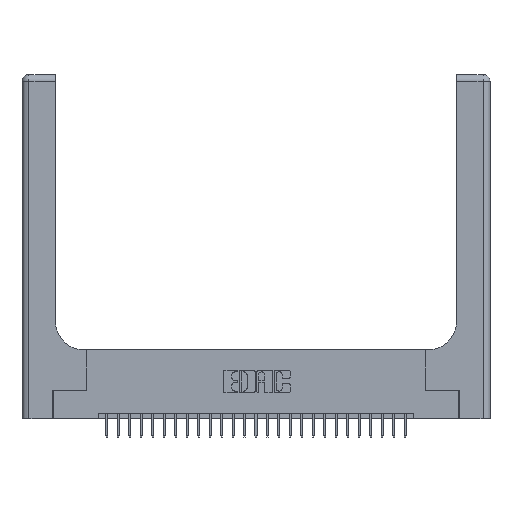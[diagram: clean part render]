
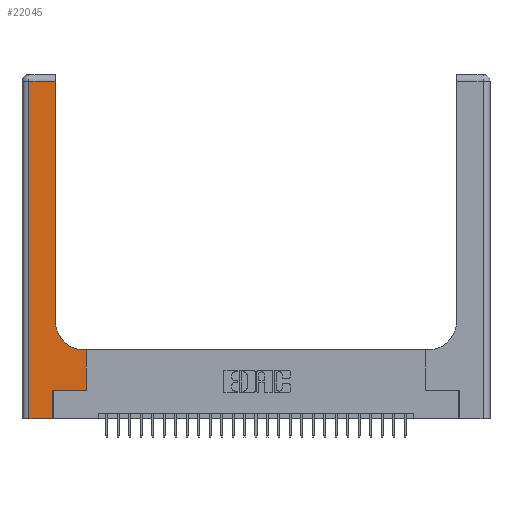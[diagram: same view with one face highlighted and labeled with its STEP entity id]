
A CAD part, top view. The second image highlights one B-rep face of the part: STEP entity #22045.
In plain terms, the highlighted planar face has unit normal (0, 0, 1).
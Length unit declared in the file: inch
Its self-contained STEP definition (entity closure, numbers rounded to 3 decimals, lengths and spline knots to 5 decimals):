
#95 = CARTESIAN_POINT ( 'NONE',  ( 0., 2.94, 0.37 ) ) ;
#157 = VECTOR ( 'NONE', #3752, 39.37008 ) ;
#340 = CARTESIAN_POINT ( 'NONE',  ( 0.5585, 0.6, 0.37 ) ) ;
#359 = EDGE_CURVE ( 'NONE', #14216, #27336, #12502, .T. ) ;
#906 = VERTEX_POINT ( 'NONE', #1702 ) ;
#1003 = ORIENTED_EDGE ( 'NONE', *, *, #15450, .T. ) ;
#1260 = AXIS2_PLACEMENT_3D ( 'NONE', #23808, #10776, #25950 ) ;
#1341 = CARTESIAN_POINT ( 'NONE',  ( 0.5415, 0.6, 0.37 ) ) ;
#1397 = ORIENTED_EDGE ( 'NONE', *, *, #9048, .T. ) ;
#1694 = CARTESIAN_POINT ( 'NONE',  ( 0.5585, 0.25, 0.37 ) ) ;
#1702 = CARTESIAN_POINT ( 'NONE',  ( 0.06, 2.94, 0.37 ) ) ;
#2161 = DIRECTION ( 'NONE',  ( -1., 0., 0. ) ) ;
#2397 = DIRECTION ( 'NONE',  ( -1., 0., 0. ) ) ;
#2763 = CARTESIAN_POINT ( 'NONE',  ( 0.06, 3., 0.37 ) ) ;
#2784 = VECTOR ( 'NONE', #6668, 39.37008 ) ;
#3312 = VERTEX_POINT ( 'NONE', #1694 ) ;
#3359 = VERTEX_POINT ( 'NONE', #10754 ) ;
#3545 = CARTESIAN_POINT ( 'NONE',  ( 0.2915, 2.94, 0.37 ) ) ;
#3582 = ORIENTED_EDGE ( 'NONE', *, *, #26707, .T. ) ;
#3752 = DIRECTION ( 'NONE',  ( 0., 1., 0. ) ) ;
#4565 = ORIENTED_EDGE ( 'NONE', *, *, #6245, .T. ) ;
#5023 = DIRECTION ( 'NONE',  ( 0., -1., 0. ) ) ;
#5375 = ORIENTED_EDGE ( 'NONE', *, *, #9801, .T. ) ;
#6245 = EDGE_CURVE ( 'NONE', #17112, #3359, #12211, .T. ) ;
#6668 = DIRECTION ( 'NONE',  ( 1., 0., 0. ) ) ;
#7651 = DIRECTION ( 'NONE',  ( 0., 1., 0. ) ) ;
#8170 = VERTEX_POINT ( 'NONE', #3545 ) ;
#8178 = EDGE_LOOP ( 'NONE', ( #24019, #5375, #8400, #12252, #4565, #1397, #3582, #14459, #1003 ) ) ;
#8400 = ORIENTED_EDGE ( 'NONE', *, *, #16380, .T. ) ;
#8518 = VECTOR ( 'NONE', #25451, 39.37008 ) ;
#8765 = LINE ( 'NONE', #19908, #2784 ) ;
#8846 = DIRECTION ( 'NONE',  ( 0., 0., -1. ) ) ;
#8853 = DIRECTION ( 'NONE',  ( 1., 0., 0. ) ) ;
#8907 = VERTEX_POINT ( 'NONE', #19254 ) ;
#9048 = EDGE_CURVE ( 'NONE', #3359, #3312, #8765, .T. ) ;
#9801 = EDGE_CURVE ( 'NONE', #8170, #906, #15629, .T. ) ;
#10754 = CARTESIAN_POINT ( 'NONE',  ( 0.269, 0.25, 0.37 ) ) ;
#10776 = DIRECTION ( 'NONE',  ( 0., 0., -1. ) ) ;
#12152 = LINE ( 'NONE', #14822, #157 ) ;
#12211 = LINE ( 'NONE', #20835, #17347 ) ;
#12252 = ORIENTED_EDGE ( 'NONE', *, *, #26951, .T. ) ;
#12502 = LINE ( 'NONE', #28477, #16931 ) ;
#13339 = VECTOR ( 'NONE', #8853, 39.37008 ) ;
#14216 = VERTEX_POINT ( 'NONE', #340 ) ;
#14459 = ORIENTED_EDGE ( 'NONE', *, *, #359, .T. ) ;
#14716 = VECTOR ( 'NONE', #5023, 39.37008 ) ;
#14768 = CIRCLE ( 'NONE', #1260, 0.25 ) ;
#14822 = CARTESIAN_POINT ( 'NONE',  ( 0.2915, 3., 0.37 ) ) ;
#15450 = EDGE_CURVE ( 'NONE', #27336, #8907, #14768, .T. ) ;
#15629 = LINE ( 'NONE', #95, #26448 ) ;
#16118 = CARTESIAN_POINT ( 'NONE',  ( 0.269, 0., 0.37 ) ) ;
#16380 = EDGE_CURVE ( 'NONE', #906, #16954, #26214, .T. ) ;
#16931 = VECTOR ( 'NONE', #26328, 39.37008 ) ;
#16954 = VERTEX_POINT ( 'NONE', #24395 ) ;
#17112 = VERTEX_POINT ( 'NONE', #16118 ) ;
#17347 = VECTOR ( 'NONE', #7651, 39.37008 ) ;
#17655 = CARTESIAN_POINT ( 'NONE',  ( 0., 0., 0.37 ) ) ;
#17997 = AXIS2_PLACEMENT_3D ( 'NONE', #26255, #8846, #2161 ) ;
#19254 = CARTESIAN_POINT ( 'NONE',  ( 0.2915, 0.85, 0.37 ) ) ;
#19876 = LINE ( 'NONE', #17655, #13339 ) ;
#19908 = CARTESIAN_POINT ( 'NONE',  ( 0.269, 0.25, 0.37 ) ) ;
#20217 = LINE ( 'NONE', #23311, #8518 ) ;
#20835 = CARTESIAN_POINT ( 'NONE',  ( 0.269, 0., 0.37 ) ) ;
#22045 = ADVANCED_FACE ( 'NONE', ( #22549 ), #28407, .F. ) ;
#22549 = FACE_OUTER_BOUND ( 'NONE', #8178, .T. ) ;
#23311 = CARTESIAN_POINT ( 'NONE',  ( 0.5585, 0.25, 0.37 ) ) ;
#23808 = CARTESIAN_POINT ( 'NONE',  ( 0.5415, 0.85, 0.37 ) ) ;
#24019 = ORIENTED_EDGE ( 'NONE', *, *, #25375, .T. ) ;
#24395 = CARTESIAN_POINT ( 'NONE',  ( 0.06, 0., 0.37 ) ) ;
#25375 = EDGE_CURVE ( 'NONE', #8907, #8170, #12152, .T. ) ;
#25451 = DIRECTION ( 'NONE',  ( 0., 1., 0. ) ) ;
#25950 = DIRECTION ( 'NONE',  ( 1., 0., 0. ) ) ;
#26214 = LINE ( 'NONE', #2763, #14716 ) ;
#26255 = CARTESIAN_POINT ( 'NONE',  ( 0., 3., 0.37 ) ) ;
#26328 = DIRECTION ( 'NONE',  ( -1., 0., 0. ) ) ;
#26448 = VECTOR ( 'NONE', #2397, 39.37008 ) ;
#26707 = EDGE_CURVE ( 'NONE', #3312, #14216, #20217, .T. ) ;
#26951 = EDGE_CURVE ( 'NONE', #16954, #17112, #19876, .T. ) ;
#27336 = VERTEX_POINT ( 'NONE', #1341 ) ;
#28407 = PLANE ( 'NONE',  #17997 ) ;
#28477 = CARTESIAN_POINT ( 'NONE',  ( 0.2915, 0.6, 0.37 ) ) ;
